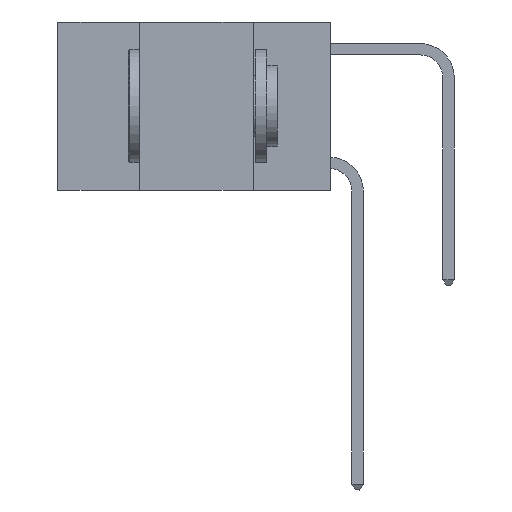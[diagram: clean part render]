
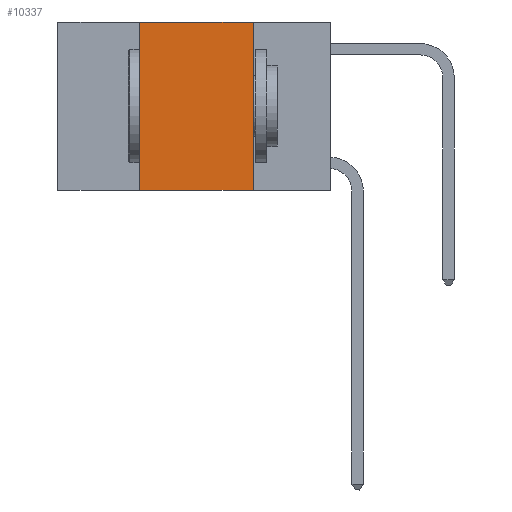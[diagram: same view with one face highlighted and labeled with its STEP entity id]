
A CAD part, left-side view. The second image highlights one B-rep face of the part: STEP entity #10337.
In plain terms, the highlighted planar face has unit normal (-1, 0, 0).
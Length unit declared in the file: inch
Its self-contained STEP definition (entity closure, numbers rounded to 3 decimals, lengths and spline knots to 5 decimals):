
#10 = CARTESIAN_POINT ( 'NONE',  ( 0., 0.42, -0.37 ) ) ;
#781 = DIRECTION ( 'NONE',  ( 0., 0., 1. ) ) ;
#1758 = EDGE_CURVE ( 'NONE', #13258, #10664, #16542, .T. ) ;
#3947 = VECTOR ( 'NONE', #14032, 39.37008 ) ;
#4232 = ORIENTED_EDGE ( 'NONE', *, *, #15607, .F. ) ;
#4250 = AXIS2_PLACEMENT_3D ( 'NONE', #14598, #6450, #15978 ) ;
#5089 = ORIENTED_EDGE ( 'NONE', *, *, #10210, .F. ) ;
#5100 = PLANE ( 'NONE',  #4250 ) ;
#5683 = VECTOR ( 'NONE', #11707, 39.37008 ) ;
#5726 = EDGE_CURVE ( 'NONE', #8582, #10664, #7109, .T. ) ;
#6101 = CARTESIAN_POINT ( 'NONE',  ( 0., 0.42, 0. ) ) ;
#6220 = LINE ( 'NONE', #6101, #8899 ) ;
#6256 = EDGE_LOOP ( 'NONE', ( #14396, #4232, #5089, #9452 ) ) ;
#6450 = DIRECTION ( 'NONE',  ( 1., 0., 0. ) ) ;
#6952 = CARTESIAN_POINT ( 'NONE',  ( 0., 0.17, 0. ) ) ;
#6965 = CARTESIAN_POINT ( 'NONE',  ( 0., 0.17, -0.37 ) ) ;
#7109 = LINE ( 'NONE', #14460, #9266 ) ;
#7651 = FACE_OUTER_BOUND ( 'NONE', #6256, .T. ) ;
#7921 = LINE ( 'NONE', #12662, #3947 ) ;
#8466 = VERTEX_POINT ( 'NONE', #10551 ) ;
#8582 = VERTEX_POINT ( 'NONE', #10 ) ;
#8899 = VECTOR ( 'NONE', #781, 39.37008 ) ;
#9266 = VECTOR ( 'NONE', #10368, 39.37008 ) ;
#9452 = ORIENTED_EDGE ( 'NONE', *, *, #5726, .T. ) ;
#10210 = EDGE_CURVE ( 'NONE', #8582, #8466, #6220, .T. ) ;
#10334 = CARTESIAN_POINT ( 'NONE',  ( 0., 0.17, 0. ) ) ;
#10337 = ADVANCED_FACE ( 'NONE', ( #7651 ), #5100, .F. ) ;
#10368 = DIRECTION ( 'NONE',  ( 0., -1., 0. ) ) ;
#10551 = CARTESIAN_POINT ( 'NONE',  ( 0., 0.42, 0. ) ) ;
#10664 = VERTEX_POINT ( 'NONE', #6965 ) ;
#11707 = DIRECTION ( 'NONE',  ( 0., 0., -1. ) ) ;
#12662 = CARTESIAN_POINT ( 'NONE',  ( 0., 0.6, 0. ) ) ;
#13258 = VERTEX_POINT ( 'NONE', #6952 ) ;
#14032 = DIRECTION ( 'NONE',  ( 0., -1., 0. ) ) ;
#14396 = ORIENTED_EDGE ( 'NONE', *, *, #1758, .F. ) ;
#14460 = CARTESIAN_POINT ( 'NONE',  ( 0., 0.6, -0.37 ) ) ;
#14598 = CARTESIAN_POINT ( 'NONE',  ( 0., 0.6, 0. ) ) ;
#15607 = EDGE_CURVE ( 'NONE', #8466, #13258, #7921, .T. ) ;
#15978 = DIRECTION ( 'NONE',  ( 0., 0., -1. ) ) ;
#16542 = LINE ( 'NONE', #10334, #5683 ) ;
